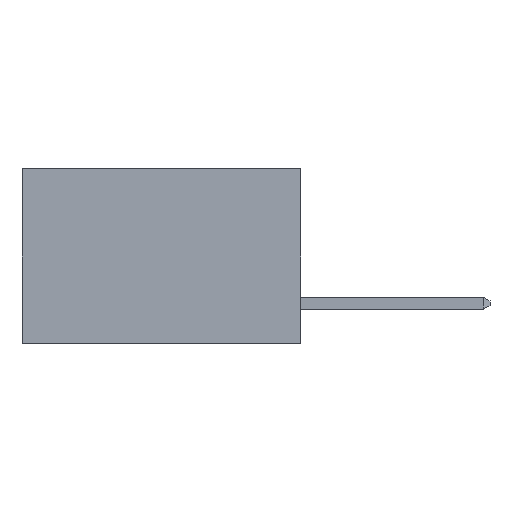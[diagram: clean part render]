
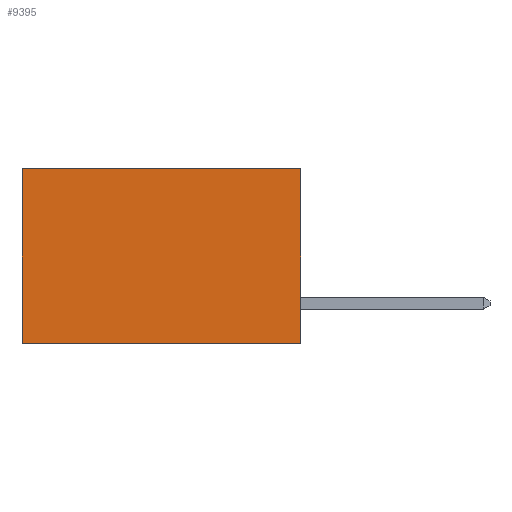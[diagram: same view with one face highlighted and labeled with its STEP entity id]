
A CAD part, left-side view. The second image highlights one B-rep face of the part: STEP entity #9395.
In plain terms, the highlighted planar face has unit normal (-1, 0, 0).
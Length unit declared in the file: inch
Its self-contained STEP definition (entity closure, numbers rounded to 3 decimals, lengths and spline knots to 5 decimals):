
#29 = ORIENTED_EDGE ( 'NONE', *, *, #2079, .T. ) ;
#803 = VERTEX_POINT ( 'NONE', #6568 ) ;
#1480 = CARTESIAN_POINT ( 'NONE',  ( 0.277, 0., -0.37 ) ) ;
#1796 = LINE ( 'NONE', #8320, #7337 ) ;
#2045 = LINE ( 'NONE', #2363, #9392 ) ;
#2079 = EDGE_CURVE ( 'NONE', #2625, #5842, #2729, .T. ) ;
#2363 = CARTESIAN_POINT ( 'NONE',  ( 0.277, 0., -0.37 ) ) ;
#2375 = FACE_OUTER_BOUND ( 'NONE', #3894, .T. ) ;
#2625 = VERTEX_POINT ( 'NONE', #4923 ) ;
#2729 = LINE ( 'NONE', #3163, #6972 ) ;
#2746 = EDGE_CURVE ( 'NONE', #8274, #803, #6637, .T. ) ;
#2820 = CARTESIAN_POINT ( 'NONE',  ( 0.277, 0., -0.37 ) ) ;
#3163 = CARTESIAN_POINT ( 'NONE',  ( 0.277, 0.59, -0.37 ) ) ;
#3185 = DIRECTION ( 'NONE',  ( 0., 0., -1. ) ) ;
#3894 = EDGE_LOOP ( 'NONE', ( #29, #4316, #8015, #6423 ) ) ;
#4259 = DIRECTION ( 'NONE',  ( 0., 1., 0. ) ) ;
#4316 = ORIENTED_EDGE ( 'NONE', *, *, #7958, .F. ) ;
#4633 = EDGE_CURVE ( 'NONE', #8274, #2625, #1796, .T. ) ;
#4896 = CARTESIAN_POINT ( 'NONE',  ( 0.277, 0.59, -0.37 ) ) ;
#4923 = CARTESIAN_POINT ( 'NONE',  ( 0.277, 0.59, 0. ) ) ;
#5377 = CARTESIAN_POINT ( 'NONE',  ( 0.277, 0., 0. ) ) ;
#5448 = DIRECTION ( 'NONE',  ( 0., 0., -1. ) ) ;
#5842 = VERTEX_POINT ( 'NONE', #4896 ) ;
#6423 = ORIENTED_EDGE ( 'NONE', *, *, #4633, .T. ) ;
#6568 = CARTESIAN_POINT ( 'NONE',  ( 0.277, 0., -0.37 ) ) ;
#6608 = AXIS2_PLACEMENT_3D ( 'NONE', #1480, #7407, #3185 ) ;
#6637 = LINE ( 'NONE', #2820, #8224 ) ;
#6831 = DIRECTION ( 'NONE',  ( 0., 0., -1. ) ) ;
#6972 = VECTOR ( 'NONE', #6831, 39.37008 ) ;
#7255 = PLANE ( 'NONE',  #6608 ) ;
#7337 = VECTOR ( 'NONE', #8427, 39.37008 ) ;
#7407 = DIRECTION ( 'NONE',  ( 1., 0., 0. ) ) ;
#7958 = EDGE_CURVE ( 'NONE', #803, #5842, #2045, .T. ) ;
#8015 = ORIENTED_EDGE ( 'NONE', *, *, #2746, .F. ) ;
#8224 = VECTOR ( 'NONE', #5448, 39.37008 ) ;
#8274 = VERTEX_POINT ( 'NONE', #5377 ) ;
#8320 = CARTESIAN_POINT ( 'NONE',  ( 0.277, 0., 0. ) ) ;
#8427 = DIRECTION ( 'NONE',  ( 0., 1., 0. ) ) ;
#9392 = VECTOR ( 'NONE', #4259, 39.37008 ) ;
#9395 = ADVANCED_FACE ( 'NONE', ( #2375 ), #7255, .F. ) ;
